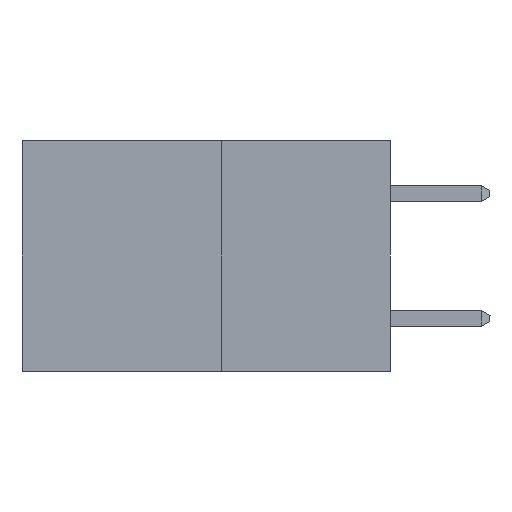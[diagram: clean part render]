
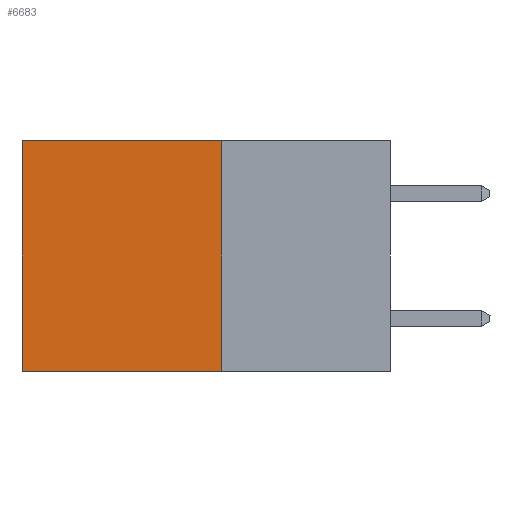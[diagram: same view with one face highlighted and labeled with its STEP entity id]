
A CAD part, left-side view. The second image highlights one B-rep face of the part: STEP entity #6683.
In plain terms, the highlighted planar face has unit normal (-1, 0, 0).
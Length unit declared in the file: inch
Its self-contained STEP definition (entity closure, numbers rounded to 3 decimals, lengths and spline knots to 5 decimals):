
#180 = EDGE_CURVE ( 'NONE', #6538, #2736, #1015, .T. ) ;
#284 = CARTESIAN_POINT ( 'NONE',  ( 0.277, 0.27, 0. ) ) ;
#315 = CARTESIAN_POINT ( 'NONE',  ( 0.277, 0.59, -0.37 ) ) ;
#359 = VECTOR ( 'NONE', #838, 39.37008 ) ;
#736 = DIRECTION ( 'NONE',  ( 1., 0., 0. ) ) ;
#838 = DIRECTION ( 'NONE',  ( 0., 1., 0. ) ) ;
#1015 = LINE ( 'NONE', #5386, #7786 ) ;
#1821 = ORIENTED_EDGE ( 'NONE', *, *, #2806, .F. ) ;
#2695 = CARTESIAN_POINT ( 'NONE',  ( 0.277, 0.59, -0.37 ) ) ;
#2736 = VERTEX_POINT ( 'NONE', #7415 ) ;
#2781 = DIRECTION ( 'NONE',  ( 0., 0., -1. ) ) ;
#2806 = EDGE_CURVE ( 'NONE', #2736, #6452, #5062, .T. ) ;
#3100 = VECTOR ( 'NONE', #3327, 39.37008 ) ;
#3246 = ORIENTED_EDGE ( 'NONE', *, *, #5675, .T. ) ;
#3270 = EDGE_LOOP ( 'NONE', ( #3246, #1821, #3433, #3544 ) ) ;
#3327 = DIRECTION ( 'NONE',  ( 0., 1., 0. ) ) ;
#3433 = ORIENTED_EDGE ( 'NONE', *, *, #180, .F. ) ;
#3544 = ORIENTED_EDGE ( 'NONE', *, *, #5628, .T. ) ;
#3852 = LINE ( 'NONE', #2695, #6899 ) ;
#4113 = DIRECTION ( 'NONE',  ( 0., 0., -1. ) ) ;
#4280 = LINE ( 'NONE', #5442, #359 ) ;
#4379 = CARTESIAN_POINT ( 'NONE',  ( 0.277, 0.27, -0.37 ) ) ;
#4480 = PLANE ( 'NONE',  #8217 ) ;
#5062 = LINE ( 'NONE', #6571, #3100 ) ;
#5386 = CARTESIAN_POINT ( 'NONE',  ( 0.277, 0.27, -0.37 ) ) ;
#5442 = CARTESIAN_POINT ( 'NONE',  ( 0.277, 0.27, 0. ) ) ;
#5628 = EDGE_CURVE ( 'NONE', #6538, #7536, #4280, .T. ) ;
#5675 = EDGE_CURVE ( 'NONE', #7536, #6452, #3852, .T. ) ;
#6006 = DIRECTION ( 'NONE',  ( 0., 0., -1. ) ) ;
#6452 = VERTEX_POINT ( 'NONE', #315 ) ;
#6531 = FACE_OUTER_BOUND ( 'NONE', #3270, .T. ) ;
#6538 = VERTEX_POINT ( 'NONE', #284 ) ;
#6571 = CARTESIAN_POINT ( 'NONE',  ( 0.277, 0.27, -0.37 ) ) ;
#6683 = ADVANCED_FACE ( 'NONE', ( #6531 ), #4480, .F. ) ;
#6772 = CARTESIAN_POINT ( 'NONE',  ( 0.277, 0.59, 0. ) ) ;
#6899 = VECTOR ( 'NONE', #2781, 39.37008 ) ;
#7415 = CARTESIAN_POINT ( 'NONE',  ( 0.277, 0.27, -0.37 ) ) ;
#7536 = VERTEX_POINT ( 'NONE', #6772 ) ;
#7786 = VECTOR ( 'NONE', #4113, 39.37008 ) ;
#8217 = AXIS2_PLACEMENT_3D ( 'NONE', #4379, #736, #6006 ) ;
